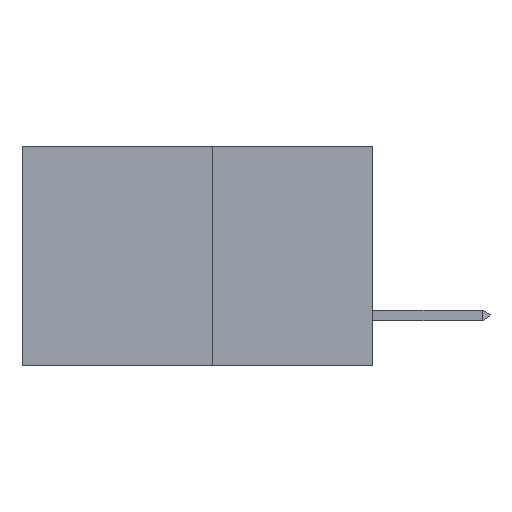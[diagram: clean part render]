
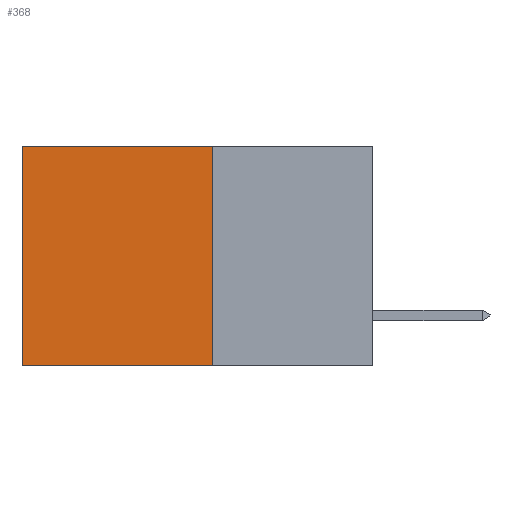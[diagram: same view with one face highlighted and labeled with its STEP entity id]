
A CAD part, left-side view. The second image highlights one B-rep face of the part: STEP entity #368.
In plain terms, the highlighted planar face has unit normal (-1, 0, 0).
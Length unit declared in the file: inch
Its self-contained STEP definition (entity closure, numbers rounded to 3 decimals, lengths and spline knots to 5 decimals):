
#368 = ADVANCED_FACE ( 'NONE', ( #20488 ), #18276, .F. ) ;
#2499 = CARTESIAN_POINT ( 'NONE',  ( 0.277, 0.59, 0. ) ) ;
#3190 = VECTOR ( 'NONE', #6370, 39.37008 ) ;
#3491 = VERTEX_POINT ( 'NONE', #2499 ) ;
#3968 = EDGE_LOOP ( 'NONE', ( #22127, #14480, #15336, #11966 ) ) ;
#4263 = CARTESIAN_POINT ( 'NONE',  ( 0.277, 0.59, -0.37 ) ) ;
#4297 = LINE ( 'NONE', #23549, #19016 ) ;
#5059 = CARTESIAN_POINT ( 'NONE',  ( 0.277, 0.59, -0.37 ) ) ;
#5412 = DIRECTION ( 'NONE',  ( 1., 0., 0. ) ) ;
#5798 = DIRECTION ( 'NONE',  ( 0., 0., -1. ) ) ;
#6370 = DIRECTION ( 'NONE',  ( 0., 1., 0. ) ) ;
#6555 = EDGE_CURVE ( 'NONE', #25466, #17950, #4297, .T. ) ;
#7834 = VERTEX_POINT ( 'NONE', #13651 ) ;
#8325 = CARTESIAN_POINT ( 'NONE',  ( 0.277, 0.27, 0. ) ) ;
#9097 = VECTOR ( 'NONE', #24221, 39.37008 ) ;
#9997 = AXIS2_PLACEMENT_3D ( 'NONE', #22420, #5412, #14128 ) ;
#10370 = LINE ( 'NONE', #15805, #24923 ) ;
#11966 = ORIENTED_EDGE ( 'NONE', *, *, #23402, .T. ) ;
#12705 = EDGE_CURVE ( 'NONE', #7834, #25466, #10370, .T. ) ;
#13651 = CARTESIAN_POINT ( 'NONE',  ( 0.277, 0.27, 0. ) ) ;
#14128 = DIRECTION ( 'NONE',  ( 0., 0., -1. ) ) ;
#14480 = ORIENTED_EDGE ( 'NONE', *, *, #6555, .F. ) ;
#14531 = LINE ( 'NONE', #8325, #3190 ) ;
#15336 = ORIENTED_EDGE ( 'NONE', *, *, #12705, .F. ) ;
#15702 = DIRECTION ( 'NONE',  ( 0., 1., 0. ) ) ;
#15805 = CARTESIAN_POINT ( 'NONE',  ( 0.277, 0.27, -0.37 ) ) ;
#17950 = VERTEX_POINT ( 'NONE', #5059 ) ;
#18276 = PLANE ( 'NONE',  #9997 ) ;
#18286 = EDGE_CURVE ( 'NONE', #3491, #17950, #24331, .T. ) ;
#19016 = VECTOR ( 'NONE', #15702, 39.37008 ) ;
#20488 = FACE_OUTER_BOUND ( 'NONE', #3968, .T. ) ;
#22127 = ORIENTED_EDGE ( 'NONE', *, *, #18286, .T. ) ;
#22420 = CARTESIAN_POINT ( 'NONE',  ( 0.277, 0.27, -0.37 ) ) ;
#23402 = EDGE_CURVE ( 'NONE', #7834, #3491, #14531, .T. ) ;
#23549 = CARTESIAN_POINT ( 'NONE',  ( 0.277, 0.27, -0.37 ) ) ;
#24221 = DIRECTION ( 'NONE',  ( 0., 0., -1. ) ) ;
#24331 = LINE ( 'NONE', #4263, #9097 ) ;
#24418 = CARTESIAN_POINT ( 'NONE',  ( 0.277, 0.27, -0.37 ) ) ;
#24923 = VECTOR ( 'NONE', #5798, 39.37008 ) ;
#25466 = VERTEX_POINT ( 'NONE', #24418 ) ;
